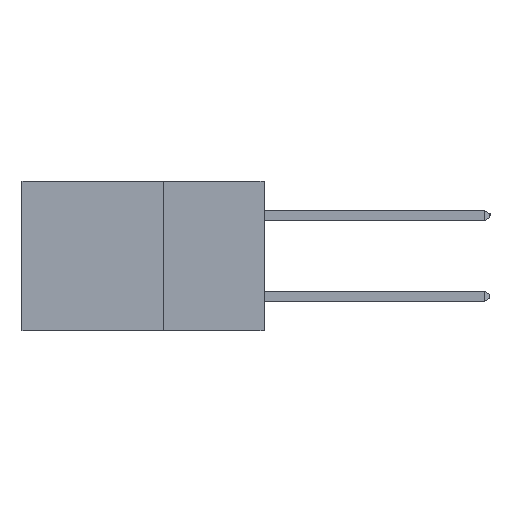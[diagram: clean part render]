
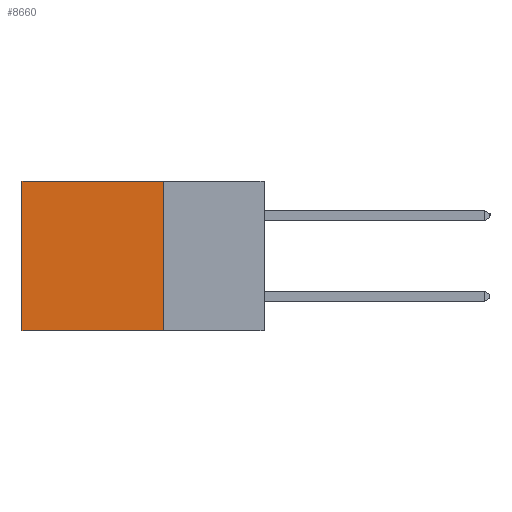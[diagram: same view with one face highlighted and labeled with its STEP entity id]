
A CAD part, left-side view. The second image highlights one B-rep face of the part: STEP entity #8660.
In plain terms, the highlighted planar face has unit normal (-1, 0, 0).
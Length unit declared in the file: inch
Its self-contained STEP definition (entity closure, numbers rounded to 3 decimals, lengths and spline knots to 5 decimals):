
#234 = EDGE_LOOP ( 'NONE', ( #1546, #8512, #4518, #10445 ) ) ;
#414 = CARTESIAN_POINT ( 'NONE',  ( 0.2615, 0.25, -0.37 ) ) ;
#458 = AXIS2_PLACEMENT_3D ( 'NONE', #1337, #2305, #4426 ) ;
#640 = EDGE_CURVE ( 'NONE', #9177, #4327, #11548, .T. ) ;
#1152 = EDGE_CURVE ( 'NONE', #9177, #5623, #7039, .T. ) ;
#1337 = CARTESIAN_POINT ( 'NONE',  ( 0.2615, 0.25, -0.37 ) ) ;
#1546 = ORIENTED_EDGE ( 'NONE', *, *, #9455, .T. ) ;
#2145 = CARTESIAN_POINT ( 'NONE',  ( 0.2615, 0.25, 0. ) ) ;
#2189 = CARTESIAN_POINT ( 'NONE',  ( 0.2615, 0.6, -0.37 ) ) ;
#2305 = DIRECTION ( 'NONE',  ( 1., 0., 0. ) ) ;
#2772 = CARTESIAN_POINT ( 'NONE',  ( 0.2615, 0.25, -0.37 ) ) ;
#3180 = VECTOR ( 'NONE', #6069, 39.37008 ) ;
#3517 = VERTEX_POINT ( 'NONE', #5703 ) ;
#4113 = DIRECTION ( 'NONE',  ( 0., 0., -1. ) ) ;
#4327 = VERTEX_POINT ( 'NONE', #7738 ) ;
#4426 = DIRECTION ( 'NONE',  ( 0., 0., -1. ) ) ;
#4449 = VECTOR ( 'NONE', #7162, 39.37008 ) ;
#4518 = ORIENTED_EDGE ( 'NONE', *, *, #640, .F. ) ;
#4623 = EDGE_CURVE ( 'NONE', #4327, #3517, #9267, .T. ) ;
#5003 = VECTOR ( 'NONE', #6698, 39.37008 ) ;
#5381 = PLANE ( 'NONE',  #458 ) ;
#5623 = VERTEX_POINT ( 'NONE', #11087 ) ;
#5703 = CARTESIAN_POINT ( 'NONE',  ( 0.2615, 0.6, -0.37 ) ) ;
#6069 = DIRECTION ( 'NONE',  ( 0., 1., 0. ) ) ;
#6698 = DIRECTION ( 'NONE',  ( 0., 0., -1. ) ) ;
#7039 = LINE ( 'NONE', #2145, #3180 ) ;
#7138 = LINE ( 'NONE', #2189, #11848 ) ;
#7162 = DIRECTION ( 'NONE',  ( 0., 1., 0. ) ) ;
#7652 = CARTESIAN_POINT ( 'NONE',  ( 0.2615, 0.25, 0. ) ) ;
#7738 = CARTESIAN_POINT ( 'NONE',  ( 0.2615, 0.25, -0.37 ) ) ;
#8512 = ORIENTED_EDGE ( 'NONE', *, *, #4623, .F. ) ;
#8660 = ADVANCED_FACE ( 'NONE', ( #12306 ), #5381, .F. ) ;
#9177 = VERTEX_POINT ( 'NONE', #7652 ) ;
#9267 = LINE ( 'NONE', #414, #4449 ) ;
#9455 = EDGE_CURVE ( 'NONE', #5623, #3517, #7138, .T. ) ;
#10445 = ORIENTED_EDGE ( 'NONE', *, *, #1152, .T. ) ;
#11087 = CARTESIAN_POINT ( 'NONE',  ( 0.2615, 0.6, 0. ) ) ;
#11548 = LINE ( 'NONE', #2772, #5003 ) ;
#11848 = VECTOR ( 'NONE', #4113, 39.37008 ) ;
#12306 = FACE_OUTER_BOUND ( 'NONE', #234, .T. ) ;
